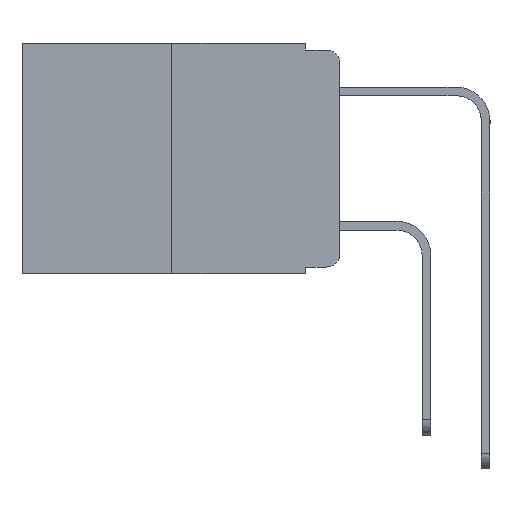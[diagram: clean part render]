
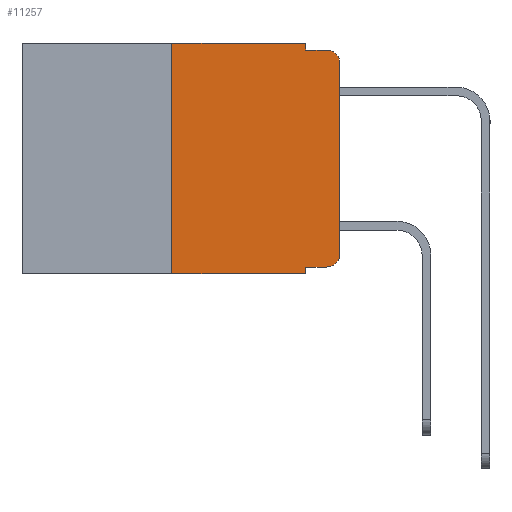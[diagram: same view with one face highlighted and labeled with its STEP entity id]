
A CAD part, left-side view. The second image highlights one B-rep face of the part: STEP entity #11257.
In plain terms, the highlighted planar face has unit normal (-1, 0, 0).
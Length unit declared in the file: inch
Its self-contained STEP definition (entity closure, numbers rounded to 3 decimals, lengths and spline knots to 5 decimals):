
#218 = LINE ( 'NONE', #15659, #12984 ) ;
#508 = DIRECTION ( 'NONE',  ( 0., -1., 0. ) ) ;
#690 = CARTESIAN_POINT ( 'NONE',  ( 0., 0., -0.03 ) ) ;
#839 = LINE ( 'NONE', #4687, #13175 ) ;
#864 = EDGE_CURVE ( 'NONE', #7708, #3586, #4239, .T. ) ;
#877 = DIRECTION ( 'NONE',  ( 1., 0., 0. ) ) ;
#1052 = CIRCLE ( 'NONE', #4978, 0.02 ) ;
#1214 = ORIENTED_EDGE ( 'NONE', *, *, #2491, .F. ) ;
#1773 = VERTEX_POINT ( 'NONE', #7958 ) ;
#2305 = CARTESIAN_POINT ( 'NONE',  ( 0., 0.25, 0. ) ) ;
#2399 = EDGE_CURVE ( 'NONE', #2985, #9145, #218, .T. ) ;
#2417 = EDGE_CURVE ( 'NONE', #9145, #1773, #3218, .T. ) ;
#2491 = EDGE_CURVE ( 'NONE', #9892, #1773, #14669, .T. ) ;
#2582 = EDGE_CURVE ( 'NONE', #15490, #9892, #839, .T. ) ;
#2608 = VECTOR ( 'NONE', #8268, 39.37008 ) ;
#2632 = EDGE_CURVE ( 'NONE', #7708, #2682, #15553, .T. ) ;
#2682 = VERTEX_POINT ( 'NONE', #4907 ) ;
#2721 = EDGE_CURVE ( 'NONE', #9464, #3586, #8071, .T. ) ;
#2722 = CARTESIAN_POINT ( 'NONE',  ( 0., 0.02, -0.03 ) ) ;
#2724 = EDGE_CURVE ( 'NONE', #9464, #7646, #14112, .T. ) ;
#2730 = EDGE_CURVE ( 'NONE', #7646, #2985, #1052, .T. ) ;
#2843 = DIRECTION ( 'NONE',  ( 0., 0., -1. ) ) ;
#2975 = ORIENTED_EDGE ( 'NONE', *, *, #2399, .T. ) ;
#2985 = VERTEX_POINT ( 'NONE', #13639 ) ;
#3177 = ORIENTED_EDGE ( 'NONE', *, *, #2582, .F. ) ;
#3218 = CIRCLE ( 'NONE', #9358, 0.02 ) ;
#3354 = CARTESIAN_POINT ( 'NONE',  ( 0., 0.473, 0. ) ) ;
#3497 = CARTESIAN_POINT ( 'NONE',  ( 0., 0.02, -0.333 ) ) ;
#3586 = VERTEX_POINT ( 'NONE', #8858 ) ;
#4029 = DIRECTION ( 'NONE',  ( 0., -1., 0. ) ) ;
#4239 = LINE ( 'NONE', #6136, #7551 ) ;
#4427 = CARTESIAN_POINT ( 'NONE',  ( 0., 0.051, -0.01 ) ) ;
#4562 = ORIENTED_EDGE ( 'NONE', *, *, #864, .T. ) ;
#4687 = CARTESIAN_POINT ( 'NONE',  ( 0., 0.051, 0. ) ) ;
#4797 = DIRECTION ( 'NONE',  ( -1., 0., 0. ) ) ;
#4907 = CARTESIAN_POINT ( 'NONE',  ( 0., 0.25, 0. ) ) ;
#4978 = AXIS2_PLACEMENT_3D ( 'NONE', #12865, #12853, #2843 ) ;
#5003 = VECTOR ( 'NONE', #13383, 39.37008 ) ;
#5231 = DIRECTION ( 'NONE',  ( 0., 0., -1. ) ) ;
#6136 = CARTESIAN_POINT ( 'NONE',  ( 0., 0.473, -0.343 ) ) ;
#6664 = ORIENTED_EDGE ( 'NONE', *, *, #2417, .T. ) ;
#6695 = ORIENTED_EDGE ( 'NONE', *, *, #2724, .T. ) ;
#7023 = CARTESIAN_POINT ( 'NONE',  ( 0., 0.473, 0. ) ) ;
#7083 = ORIENTED_EDGE ( 'NONE', *, *, #2730, .T. ) ;
#7375 = CARTESIAN_POINT ( 'NONE',  ( 0., 0.051, 0. ) ) ;
#7551 = VECTOR ( 'NONE', #508, 39.37008 ) ;
#7646 = VERTEX_POINT ( 'NONE', #3497 ) ;
#7681 = VECTOR ( 'NONE', #4029, 39.37008 ) ;
#7708 = VERTEX_POINT ( 'NONE', #9695 ) ;
#7958 = CARTESIAN_POINT ( 'NONE',  ( 0., 0.02, -0.01 ) ) ;
#8071 = LINE ( 'NONE', #14070, #11666 ) ;
#8268 = DIRECTION ( 'NONE',  ( 0., -1., 0. ) ) ;
#8641 = CARTESIAN_POINT ( 'NONE',  ( 0., 0.051, -0.333 ) ) ;
#8858 = CARTESIAN_POINT ( 'NONE',  ( 0., 0.051, -0.343 ) ) ;
#9145 = VERTEX_POINT ( 'NONE', #690 ) ;
#9358 = AXIS2_PLACEMENT_3D ( 'NONE', #2722, #4797, #5231 ) ;
#9464 = VERTEX_POINT ( 'NONE', #8641 ) ;
#9550 = DIRECTION ( 'NONE',  ( 0., 0., -1. ) ) ;
#9695 = CARTESIAN_POINT ( 'NONE',  ( 0., 0.25, -0.343 ) ) ;
#9892 = VERTEX_POINT ( 'NONE', #4427 ) ;
#9957 = VECTOR ( 'NONE', #14730, 39.37008 ) ;
#10113 = ORIENTED_EDGE ( 'NONE', *, *, #14026, .F. ) ;
#10127 = ORIENTED_EDGE ( 'NONE', *, *, #2721, .F. ) ;
#11257 = ADVANCED_FACE ( 'NONE', ( #12080 ), #14351, .F. ) ;
#11666 = VECTOR ( 'NONE', #13809, 39.37008 ) ;
#12080 = FACE_OUTER_BOUND ( 'NONE', #13423, .T. ) ;
#12380 = LINE ( 'NONE', #7023, #2608 ) ;
#12853 = DIRECTION ( 'NONE',  ( -1., 0., 0. ) ) ;
#12865 = CARTESIAN_POINT ( 'NONE',  ( 0., 0.02, -0.313 ) ) ;
#12984 = VECTOR ( 'NONE', #15225, 39.37008 ) ;
#13175 = VECTOR ( 'NONE', #13754, 39.37008 ) ;
#13383 = DIRECTION ( 'NONE',  ( 0., -1., 0. ) ) ;
#13423 = EDGE_LOOP ( 'NONE', ( #2975, #6664, #1214, #3177, #10113, #14450, #4562, #10127, #6695, #7083 ) ) ;
#13639 = CARTESIAN_POINT ( 'NONE',  ( 0., 0., -0.313 ) ) ;
#13754 = DIRECTION ( 'NONE',  ( 0., 0., -1. ) ) ;
#13809 = DIRECTION ( 'NONE',  ( 0., 0., -1. ) ) ;
#14019 = CARTESIAN_POINT ( 'NONE',  ( 0., 0.051, -0.333 ) ) ;
#14026 = EDGE_CURVE ( 'NONE', #2682, #15490, #12380, .T. ) ;
#14070 = CARTESIAN_POINT ( 'NONE',  ( 0., 0.051, 0. ) ) ;
#14112 = LINE ( 'NONE', #14019, #7681 ) ;
#14351 = PLANE ( 'NONE',  #14606 ) ;
#14450 = ORIENTED_EDGE ( 'NONE', *, *, #2632, .F. ) ;
#14606 = AXIS2_PLACEMENT_3D ( 'NONE', #3354, #877, #9550 ) ;
#14617 = CARTESIAN_POINT ( 'NONE',  ( 0., 0.051, -0.01 ) ) ;
#14669 = LINE ( 'NONE', #14617, #5003 ) ;
#14730 = DIRECTION ( 'NONE',  ( 0., 0., 1. ) ) ;
#15225 = DIRECTION ( 'NONE',  ( 0., 0., 1. ) ) ;
#15490 = VERTEX_POINT ( 'NONE', #7375 ) ;
#15553 = LINE ( 'NONE', #2305, #9957 ) ;
#15659 = CARTESIAN_POINT ( 'NONE',  ( 0., 0., 0. ) ) ;
